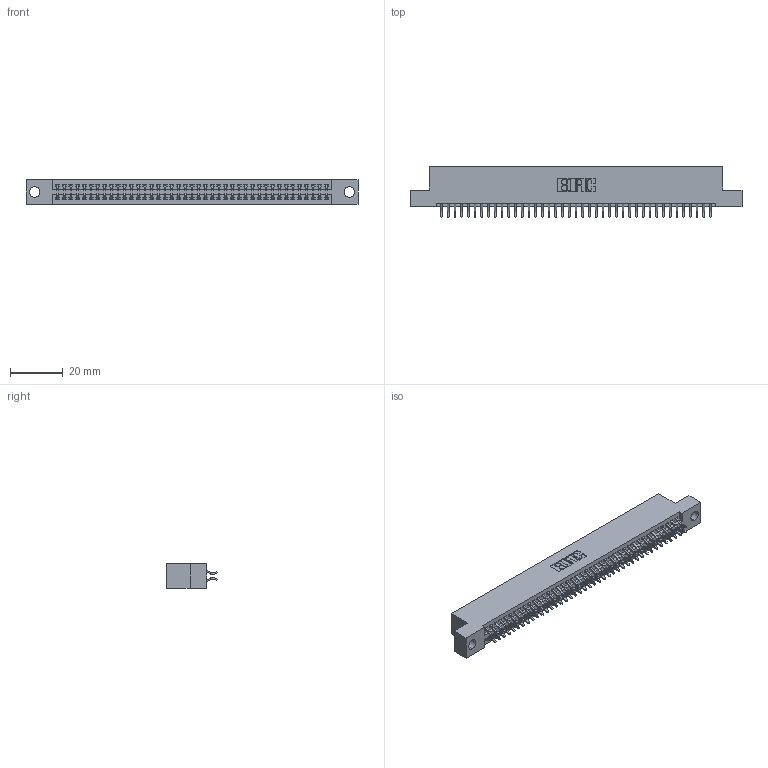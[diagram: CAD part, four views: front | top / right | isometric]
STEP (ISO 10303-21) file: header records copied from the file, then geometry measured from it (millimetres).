
FILE_DESCRIPTION (( 'STEP AP203' ), '1' );
FILE_NAME ('345-082-556-204.STEP', '2018-10-03T23:07:29', ( '' ), ( '' ), 'SwSTEP 2.0', 'SolidWorks 2016', '' );
FILE_SCHEMA (( 'CONFIG_CONTROL_DESIGN' ));
Length unit declared in the file: inch
Products named in the file (3): 345-292-001_556 Tail; 345-082-556-204; 345 Part_Flush Mounting Lugs - 0.156 Dia-TH
Assembly tree (83 placements, depth 2):
  345-082-556-204
    345 Part_Flush Mounting Lugs - 0.156 Dia-TH
    345-292-001_556 Tail  x82
Bounding box: 125.35 x 19.24 x 9.4 mm (x, y, z)
Volume: 12076.1 mm3; surface area: 17574.6 mm2
Topology: 83 solids, 83 shells, 4718 faces, 14035 edges, 9246 vertices
Faces by surface type: plane 3114, cylinder 1604
Entity records: 32527 total; most frequent: CARTESIAN_POINT 5468, ORIENTED_EDGE 5390, DIRECTION 4811, EDGE_CURVE 2695, LINE 2391, VECTOR 2391, VERTEX_POINT 1794, AXIS2_PLACEMENT_3D 1210
